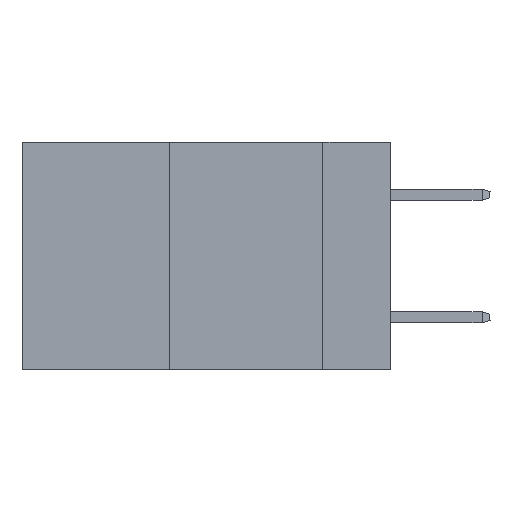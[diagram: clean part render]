
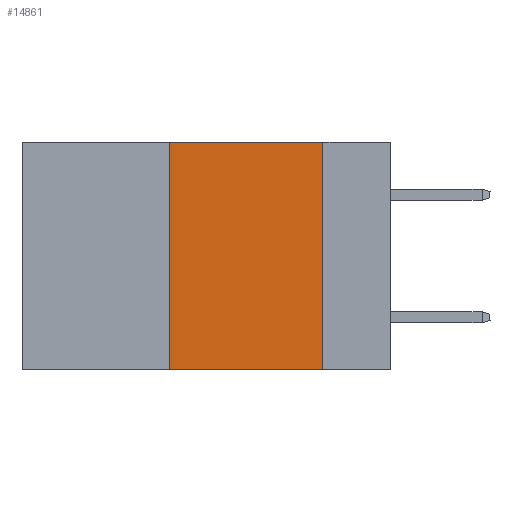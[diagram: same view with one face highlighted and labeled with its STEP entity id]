
A CAD part, left-side view. The second image highlights one B-rep face of the part: STEP entity #14861.
In plain terms, the highlighted planar face has unit normal (-1, 0, 0).
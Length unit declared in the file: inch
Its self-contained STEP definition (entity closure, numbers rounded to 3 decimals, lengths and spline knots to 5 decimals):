
#588 = EDGE_CURVE ( 'NONE', #15633, #16476, #23898, .T. ) ;
#3162 = CARTESIAN_POINT ( 'NONE',  ( 0., 0.6, -0.37 ) ) ;
#3611 = CARTESIAN_POINT ( 'NONE',  ( 0., 0.11, 0. ) ) ;
#4074 = VECTOR ( 'NONE', #20023, 39.37008 ) ;
#4258 = DIRECTION ( 'NONE',  ( 0., -1., 0. ) ) ;
#5697 = CARTESIAN_POINT ( 'NONE',  ( 0., 0.11, -0.37 ) ) ;
#5707 = EDGE_CURVE ( 'NONE', #15633, #9693, #22391, .T. ) ;
#5902 = PLANE ( 'NONE',  #33242 ) ;
#9377 = ORIENTED_EDGE ( 'NONE', *, *, #5707, .T. ) ;
#9693 = VERTEX_POINT ( 'NONE', #5697 ) ;
#9763 = VECTOR ( 'NONE', #4258, 39.37008 ) ;
#11280 = FACE_OUTER_BOUND ( 'NONE', #30287, .T. ) ;
#11826 = LINE ( 'NONE', #28119, #9763 ) ;
#12030 = DIRECTION ( 'NONE',  ( 0., 0., 1. ) ) ;
#13694 = DIRECTION ( 'NONE',  ( 0., 0., -1. ) ) ;
#13962 = CARTESIAN_POINT ( 'NONE',  ( 0., 0.36, -0.37 ) ) ;
#14648 = DIRECTION ( 'NONE',  ( 0., 0., -1. ) ) ;
#14861 = ADVANCED_FACE ( 'NONE', ( #11280 ), #5902, .F. ) ;
#15633 = VERTEX_POINT ( 'NONE', #13962 ) ;
#15651 = CARTESIAN_POINT ( 'NONE',  ( 0., 0.11, 0. ) ) ;
#16476 = VERTEX_POINT ( 'NONE', #28474 ) ;
#18034 = VECTOR ( 'NONE', #12030, 39.37008 ) ;
#18471 = VECTOR ( 'NONE', #14648, 39.37008 ) ;
#19280 = DIRECTION ( 'NONE',  ( 1., 0., 0. ) ) ;
#20023 = DIRECTION ( 'NONE',  ( 0., -1., 0. ) ) ;
#22093 = CARTESIAN_POINT ( 'NONE',  ( 0., 0.6, 0. ) ) ;
#22390 = ORIENTED_EDGE ( 'NONE', *, *, #588, .F. ) ;
#22391 = LINE ( 'NONE', #3162, #4074 ) ;
#23898 = LINE ( 'NONE', #33481, #18034 ) ;
#24259 = EDGE_CURVE ( 'NONE', #27606, #9693, #32654, .T. ) ;
#25475 = ORIENTED_EDGE ( 'NONE', *, *, #27441, .F. ) ;
#27441 = EDGE_CURVE ( 'NONE', #16476, #27606, #11826, .T. ) ;
#27606 = VERTEX_POINT ( 'NONE', #15651 ) ;
#28119 = CARTESIAN_POINT ( 'NONE',  ( 0., 0.6, 0. ) ) ;
#28474 = CARTESIAN_POINT ( 'NONE',  ( 0., 0.36, 0. ) ) ;
#30287 = EDGE_LOOP ( 'NONE', ( #30701, #25475, #22390, #9377 ) ) ;
#30701 = ORIENTED_EDGE ( 'NONE', *, *, #24259, .F. ) ;
#32654 = LINE ( 'NONE', #3611, #18471 ) ;
#33242 = AXIS2_PLACEMENT_3D ( 'NONE', #22093, #19280, #13694 ) ;
#33481 = CARTESIAN_POINT ( 'NONE',  ( 0., 0.36, 0. ) ) ;
